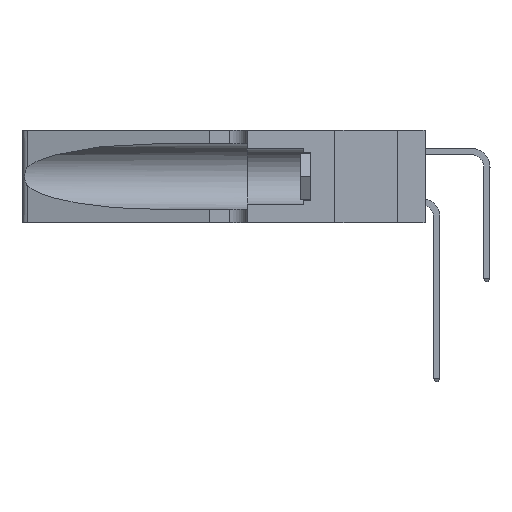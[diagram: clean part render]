
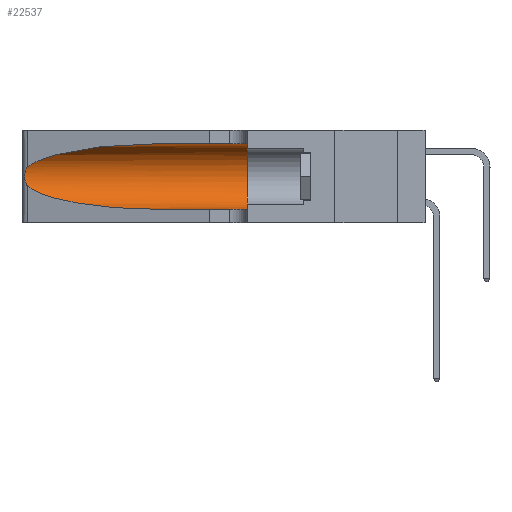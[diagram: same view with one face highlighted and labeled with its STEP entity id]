
A CAD part, left-side view. The second image highlights one B-rep face of the part: STEP entity #22537.
In plain terms, the highlighted cylindrical face has radius 3.308 mm (diameter 6.617 mm), a partial arc.
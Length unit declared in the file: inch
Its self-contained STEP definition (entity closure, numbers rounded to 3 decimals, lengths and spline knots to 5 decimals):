
#471 = CIRCLE ( 'NONE', #23508, 0.13025 ) ;
#1532 = ORIENTED_EDGE ( 'NONE', *, *, #7351, .T. ) ;
#1676 = LINE ( 'NONE', #26299, #15555 ) ;
#2079 = CARTESIAN_POINT ( 'NONE',  ( 0.26075, 1.23896, 0.178 ) ) ;
#2144 = B_SPLINE_CURVE_WITH_KNOTS ( 'NONE', 3,
 ( #38254, #20299, #35633, #11184, #26809, #20699, #8488, #2079, #8213, #29856, #29573, #11324, #5290, #36155 ),
 .UNSPECIFIED., .F., .F.,
 ( 4, 2, 2, 2, 2, 2, 4 ),
 ( 0., 0.00027, 0.00053, 0.00107, 0.0016, 0.00187, 0.00214 ),
 .UNSPECIFIED. ) ;
#2519 = VERTEX_POINT ( 'NONE', #24625 ) ;
#2878 = EDGE_CURVE ( 'NONE', #2519, #26517, #471, .T. ) ;
#3063 = EDGE_CURVE ( 'NONE', #17596, #26517, #9575, .T. ) ;
#4844 = CARTESIAN_POINT ( 'NONE',  ( 0.25487, 1.22718, 0.22369 ) ) ;
#5290 = CARTESIAN_POINT ( 'NONE',  ( 0.25555, 1.22993, 0.14849 ) ) ;
#6715 = VERTEX_POINT ( 'NONE', #16089 ) ;
#6816 = CARTESIAN_POINT ( 'NONE',  ( 0.25487, 1.22718, 0.14631 ) ) ;
#7351 = EDGE_CURVE ( 'NONE', #14192, #17596, #38848, .T. ) ;
#7366 = ORIENTED_EDGE ( 'NONE', *, *, #30589, .T. ) ;
#8213 = CARTESIAN_POINT ( 'NONE',  ( 0.26017, 1.23833, 0.17102 ) ) ;
#8488 = CARTESIAN_POINT ( 'NONE',  ( 0.26075, 1.23896, 0.19203 ) ) ;
#8644 = VECTOR ( 'NONE', #39300, 39.37008 ) ;
#9575 = LINE ( 'NONE', #20938, #8644 ) ;
#9658 = CARTESIAN_POINT ( 'NONE',  ( 0.2373, 1.15595, 0.28018 ) ) ;
#11184 = CARTESIAN_POINT ( 'NONE',  ( 0.25787, 1.23484, 0.2124 ) ) ;
#11324 = CARTESIAN_POINT ( 'NONE',  ( 0.25639, 1.23186, 0.15144 ) ) ;
#11350 = ORIENTED_EDGE ( 'NONE', *, *, #3063, .T. ) ;
#11489 = ORIENTED_EDGE ( 'NONE', *, *, #2878, .F. ) ;
#11532 = EDGE_CURVE ( 'NONE', #30343, #2519, #1676, .T. ) ;
#11759 = CARTESIAN_POINT ( 'NONE',  ( 0.1305, 0.72297, 0.05475 ) ) ;
#13170 = CARTESIAN_POINT ( 'NONE',  ( 0.1305, 0.72297, 0.05475 ) ) ;
#14192 = VERTEX_POINT ( 'NONE', #6816 ) ;
#15555 = VECTOR ( 'NONE', #23519, 39.37008 ) ;
#16089 = CARTESIAN_POINT ( 'NONE',  ( 0.25487, 1.22718, 0.22369 ) ) ;
#16503 = EDGE_CURVE ( 'NONE', #30343, #6715, #33006, .T. ) ;
#16516 = EDGE_LOOP ( 'NONE', ( #20869, #7366, #1532, #11350, #11489, #35501 ) ) ;
#16777 = FACE_OUTER_BOUND ( 'NONE', #16516, .T. ) ;
#17504 = CARTESIAN_POINT ( 'NONE',  ( 0.18966, 0.96281, 0.05475 ) ) ;
#17596 = VERTEX_POINT ( 'NONE', #13170 ) ;
#17868 = CARTESIAN_POINT ( 'NONE',  ( 0.18966, 0.96281, 0.31525 ) ) ;
#18401 = DIRECTION ( 'NONE',  ( 0., 0., 1. ) ) ;
#18598 = CARTESIAN_POINT ( 'NONE',  ( 0.1305, 0.35, 0.05475 ) ) ;
#20299 = CARTESIAN_POINT ( 'NONE',  ( 0.25555, 1.22994, 0.2215 ) ) ;
#20699 = CARTESIAN_POINT ( 'NONE',  ( 0.26018, 1.23835, 0.19895 ) ) ;
#20869 = ORIENTED_EDGE ( 'NONE', *, *, #16503, .T. ) ;
#20938 = CARTESIAN_POINT ( 'NONE',  ( 0.1305, 1.61858, 0.05475 ) ) ;
#22537 = ADVANCED_FACE ( 'NONE', ( #16777 ), #26302, .F. ) ;
#23508 = AXIS2_PLACEMENT_3D ( 'NONE', #39486, #39349, #18401 ) ;
#23519 = DIRECTION ( 'NONE',  ( 0., -1., 0. ) ) ;
#24423 = CARTESIAN_POINT ( 'NONE',  ( 0.1305, 1.61858, 0.185 ) ) ;
#24625 = CARTESIAN_POINT ( 'NONE',  ( 0.1305, 0.35, 0.31525 ) ) ;
#26299 = CARTESIAN_POINT ( 'NONE',  ( 0.1305, 1.61858, 0.31525 ) ) ;
#26302 = CYLINDRICAL_SURFACE ( 'NONE', #27332, 0.13025 ) ;
#26517 = VERTEX_POINT ( 'NONE', #18598 ) ;
#26574 = CARTESIAN_POINT ( 'NONE',  ( 0.2373, 1.15595, 0.08982 ) ) ;
#26809 = CARTESIAN_POINT ( 'NONE',  ( 0.25854, 1.2359, 0.20912 ) ) ;
#27332 = AXIS2_PLACEMENT_3D ( 'NONE', #24423, #27597, #33618 ) ;
#27581 = CARTESIAN_POINT ( 'NONE',  ( 0.1305, 0.72297, 0.31525 ) ) ;
#27597 = DIRECTION ( 'NONE',  ( 0., -1., 0. ) ) ;
#28400 = CARTESIAN_POINT ( 'NONE',  ( 0.1305, 0.72297, 0.31525 ) ) ;
#29573 = CARTESIAN_POINT ( 'NONE',  ( 0.25789, 1.23486, 0.15765 ) ) ;
#29755 = CARTESIAN_POINT ( 'NONE',  ( 0.25487, 1.22718, 0.14631 ) ) ;
#29856 = CARTESIAN_POINT ( 'NONE',  ( 0.25856, 1.23593, 0.16098 ) ) ;
#30343 = VERTEX_POINT ( 'NONE', #28400 ) ;
#30589 = EDGE_CURVE ( 'NONE', #6715, #14192, #2144, .T. ) ;
#33006 =( BOUNDED_CURVE ( )  B_SPLINE_CURVE ( 3, ( #27581, #17868, #9658, #4844 ),
 .UNSPECIFIED., .F., .F. ) 
 B_SPLINE_CURVE_WITH_KNOTS ( ( 4, 4 ),
 ( 1.5708, 2.84003 ),
 .UNSPECIFIED. ) 
 CURVE ( )  GEOMETRIC_REPRESENTATION_ITEM ( )  RATIONAL_B_SPLINE_CURVE ( ( 1., 0.87, 0.87, 1. ) ) 
 REPRESENTATION_ITEM ( '' )  );
#33618 = DIRECTION ( 'NONE',  ( 0., 0., -1. ) ) ;
#35501 = ORIENTED_EDGE ( 'NONE', *, *, #11532, .F. ) ;
#35633 = CARTESIAN_POINT ( 'NONE',  ( 0.25639, 1.23184, 0.21858 ) ) ;
#36155 = CARTESIAN_POINT ( 'NONE',  ( 0.25487, 1.22718, 0.14631 ) ) ;
#38254 = CARTESIAN_POINT ( 'NONE',  ( 0.25487, 1.22718, 0.22369 ) ) ;
#38848 =( BOUNDED_CURVE ( )  B_SPLINE_CURVE ( 3, ( #29755, #26574, #17504, #11759 ),
 .UNSPECIFIED., .F., .T. ) 
 B_SPLINE_CURVE_WITH_KNOTS ( ( 4, 4 ),
 ( 3.44316, 4.71239 ),
 .UNSPECIFIED. ) 
 CURVE ( )  GEOMETRIC_REPRESENTATION_ITEM ( )  RATIONAL_B_SPLINE_CURVE ( ( 1., 0.87, 0.87, 1. ) ) 
 REPRESENTATION_ITEM ( '' )  );
#39300 = DIRECTION ( 'NONE',  ( 0., -1., 0. ) ) ;
#39349 = DIRECTION ( 'NONE',  ( 0., 1., 0. ) ) ;
#39486 = CARTESIAN_POINT ( 'NONE',  ( 0.1305, 0.35, 0.185 ) ) ;
